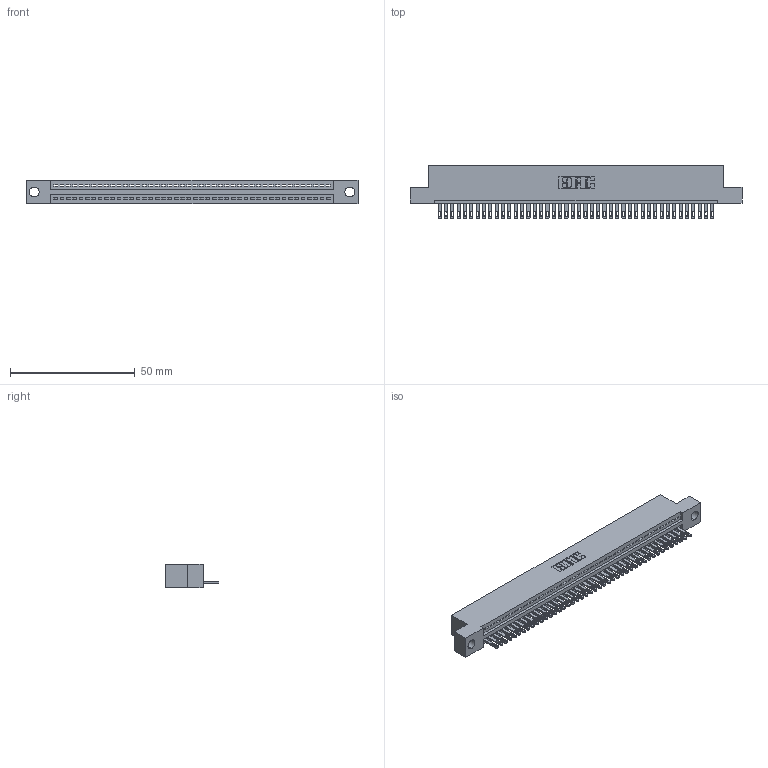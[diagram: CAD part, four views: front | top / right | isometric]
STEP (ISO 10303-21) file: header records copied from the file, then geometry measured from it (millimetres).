
FILE_DESCRIPTION (( 'STEP AP203' ), '1' );
FILE_NAME ('345-044-500-104.STEP', '2018-09-08T07:57:41', ( '' ), ( '' ), 'SwSTEP 2.0', 'SolidWorks 2016', '' );
FILE_SCHEMA (( 'CONFIG_CONTROL_DESIGN' ));
Length unit declared in the file: inch
Products named in the file (3): 345 Part_Flush Mounting Lugs - 0.156 Dia-TH; 345-292-001_345-293-100; 345-044-500-104
Assembly tree (45 placements, depth 2):
  345-044-500-104
    345 Part_Flush Mounting Lugs - 0.156 Dia-TH
    345-292-001_345-293-100  x44
Bounding box: 132.97 x 21.51 x 9.4 mm (x, y, z)
Volume: 12585.3 mm3; surface area: 16659.5 mm2
Topology: 45 solids, 45 shells, 2502 faces, 7733 edges, 5154 vertices
Faces by surface type: plane 1576, cylinder 926
Entity records: 32779 total; most frequent: CARTESIAN_POINT 5684, ORIENTED_EDGE 5662, DIRECTION 4963, EDGE_CURVE 2831, VECTOR 2519, LINE 2519, VERTEX_POINT 1886, AXIS2_PLACEMENT_3D 1222
